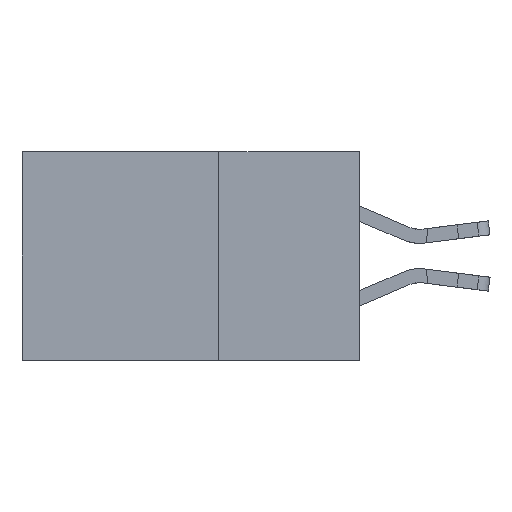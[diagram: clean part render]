
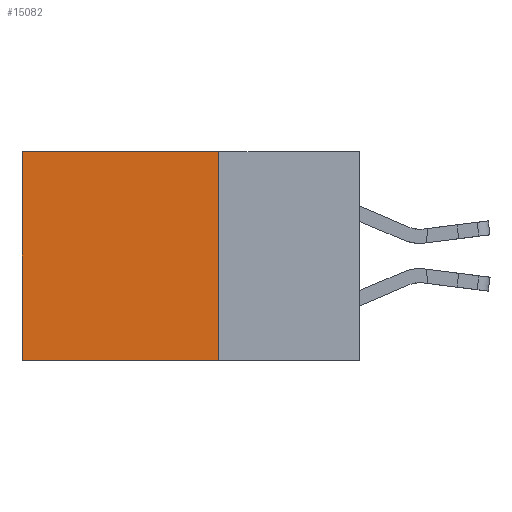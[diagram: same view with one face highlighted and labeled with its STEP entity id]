
A CAD part, left-side view. The second image highlights one B-rep face of the part: STEP entity #15082.
In plain terms, the highlighted planar face has unit normal (-1, 0, 0).
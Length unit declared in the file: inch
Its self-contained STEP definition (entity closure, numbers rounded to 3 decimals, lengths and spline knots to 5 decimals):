
#1292 = EDGE_CURVE ( 'NONE', #6854, #13206, #25636, .T. ) ;
#2066 = AXIS2_PLACEMENT_3D ( 'NONE', #4863, #24028, #11014 ) ;
#2650 = CARTESIAN_POINT ( 'NONE',  ( 0.2875, 0.25, 0. ) ) ;
#4863 = CARTESIAN_POINT ( 'NONE',  ( 0.2875, 0.25, 0. ) ) ;
#6269 = CARTESIAN_POINT ( 'NONE',  ( 0.2875, 0.6, 0. ) ) ;
#6728 = EDGE_CURVE ( 'NONE', #13206, #11111, #7748, .T. ) ;
#6854 = VERTEX_POINT ( 'NONE', #2650 ) ;
#6901 = CARTESIAN_POINT ( 'NONE',  ( 0.2875, 0.25, 0. ) ) ;
#6971 = EDGE_LOOP ( 'NONE', ( #9276, #16239, #15310, #7645 ) ) ;
#7645 = ORIENTED_EDGE ( 'NONE', *, *, #22918, .T. ) ;
#7748 = LINE ( 'NONE', #17448, #25715 ) ;
#7885 = VECTOR ( 'NONE', #15315, 39.37008 ) ;
#7886 = DIRECTION ( 'NONE',  ( 0., 0., -1. ) ) ;
#8345 = EDGE_CURVE ( 'NONE', #10069, #11111, #16444, .T. ) ;
#9276 = ORIENTED_EDGE ( 'NONE', *, *, #8345, .T. ) ;
#10069 = VERTEX_POINT ( 'NONE', #6269 ) ;
#11014 = DIRECTION ( 'NONE',  ( 0., 0., -1. ) ) ;
#11027 = VECTOR ( 'NONE', #23995, 39.37008 ) ;
#11111 = VERTEX_POINT ( 'NONE', #16151 ) ;
#13206 = VERTEX_POINT ( 'NONE', #15207 ) ;
#15082 = ADVANCED_FACE ( 'NONE', ( #15563 ), #21868, .F. ) ;
#15207 = CARTESIAN_POINT ( 'NONE',  ( 0.2875, 0.25, -0.37 ) ) ;
#15310 = ORIENTED_EDGE ( 'NONE', *, *, #1292, .F. ) ;
#15315 = DIRECTION ( 'NONE',  ( 0., 1., 0. ) ) ;
#15563 = FACE_OUTER_BOUND ( 'NONE', #6971, .T. ) ;
#16151 = CARTESIAN_POINT ( 'NONE',  ( 0.2875, 0.6, -0.37 ) ) ;
#16239 = ORIENTED_EDGE ( 'NONE', *, *, #6728, .F. ) ;
#16444 = LINE ( 'NONE', #27204, #24267 ) ;
#17448 = CARTESIAN_POINT ( 'NONE',  ( 0.2875, 0.25, -0.37 ) ) ;
#18704 = LINE ( 'NONE', #6901, #7885 ) ;
#20104 = CARTESIAN_POINT ( 'NONE',  ( 0.2875, 0.25, 0. ) ) ;
#21735 = DIRECTION ( 'NONE',  ( 0., 1., 0. ) ) ;
#21868 = PLANE ( 'NONE',  #2066 ) ;
#22918 = EDGE_CURVE ( 'NONE', #6854, #10069, #18704, .T. ) ;
#23995 = DIRECTION ( 'NONE',  ( 0., 0., -1. ) ) ;
#24028 = DIRECTION ( 'NONE',  ( 1., 0., 0. ) ) ;
#24267 = VECTOR ( 'NONE', #7886, 39.37008 ) ;
#25636 = LINE ( 'NONE', #20104, #11027 ) ;
#25715 = VECTOR ( 'NONE', #21735, 39.37008 ) ;
#27204 = CARTESIAN_POINT ( 'NONE',  ( 0.2875, 0.6, 0. ) ) ;
